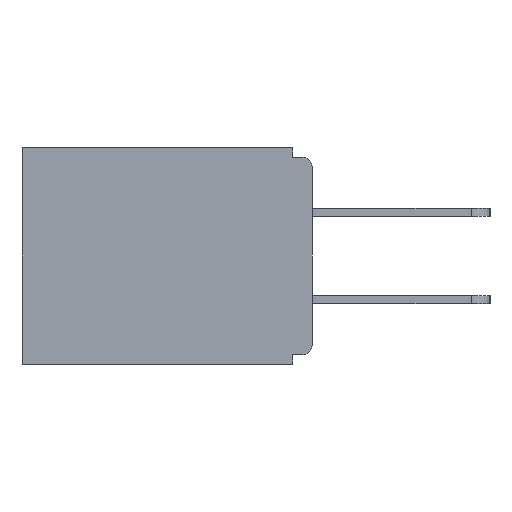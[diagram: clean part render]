
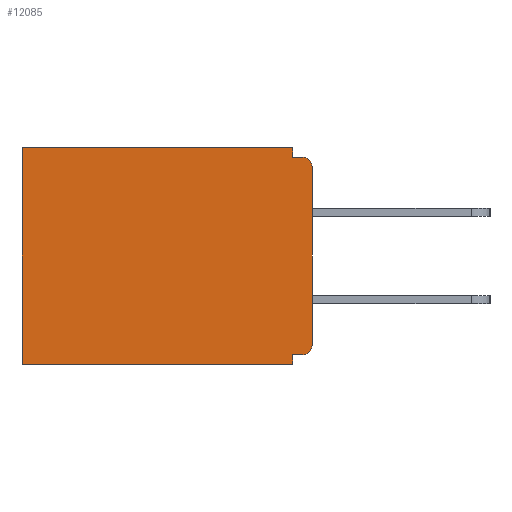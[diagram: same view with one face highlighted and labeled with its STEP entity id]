
A CAD part, left-side view. The second image highlights one B-rep face of the part: STEP entity #12085.
In plain terms, the highlighted planar face has unit normal (-1, 0, 0).
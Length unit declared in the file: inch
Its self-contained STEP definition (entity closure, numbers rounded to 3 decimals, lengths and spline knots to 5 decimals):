
#269 = ORIENTED_EDGE ( 'NONE', *, *, #14848, .F. ) ;
#725 = AXIS2_PLACEMENT_3D ( 'NONE', #785, #15022, #5420 ) ;
#785 = CARTESIAN_POINT ( 'NONE',  ( 0.298, 0.015, -0.03 ) ) ;
#823 = VECTOR ( 'NONE', #6712, 39.37008 ) ;
#898 = EDGE_CURVE ( 'NONE', #6197, #3613, #15210, .T. ) ;
#1183 = LINE ( 'NONE', #10388, #823 ) ;
#1214 = EDGE_CURVE ( 'NONE', #7799, #14307, #14885, .T. ) ;
#1244 = ORIENTED_EDGE ( 'NONE', *, *, #13400, .F. ) ;
#1270 = AXIS2_PLACEMENT_3D ( 'NONE', #12982, #9549, #7104 ) ;
#1439 = DIRECTION ( 'NONE',  ( 0., 0., -1. ) ) ;
#1534 = VERTEX_POINT ( 'NONE', #3962 ) ;
#1569 = EDGE_LOOP ( 'NONE', ( #6287, #1244, #14124, #11355, #6634, #13552, #6143, #15362, #12694, #269 ) ) ;
#1958 = VERTEX_POINT ( 'NONE', #3737 ) ;
#2016 = DIRECTION ( 'NONE',  ( 0., 0., -1. ) ) ;
#2273 = CARTESIAN_POINT ( 'NONE',  ( 0.298, 0.46, 0. ) ) ;
#2879 = EDGE_CURVE ( 'NONE', #6197, #12429, #9431, .T. ) ;
#2928 = LINE ( 'NONE', #14423, #4573 ) ;
#3182 = DIRECTION ( 'NONE',  ( 0., 1., 0. ) ) ;
#3613 = VERTEX_POINT ( 'NONE', #11995 ) ;
#3727 = CARTESIAN_POINT ( 'NONE',  ( 0.298, 0.015, -0.313 ) ) ;
#3737 = CARTESIAN_POINT ( 'NONE',  ( 0.298, 0., -0.313 ) ) ;
#3962 = CARTESIAN_POINT ( 'NONE',  ( 0.298, 0., -0.03 ) ) ;
#4268 = CARTESIAN_POINT ( 'NONE',  ( 0.298, 0.031, -0.328 ) ) ;
#4573 = VECTOR ( 'NONE', #7696, 39.37008 ) ;
#4644 = EDGE_CURVE ( 'NONE', #5984, #1958, #10282, .T. ) ;
#4909 = DIRECTION ( 'NONE',  ( -1., 0., 0. ) ) ;
#5175 = DIRECTION ( 'NONE',  ( 0., 1., 0. ) ) ;
#5420 = DIRECTION ( 'NONE',  ( 0., 0., -1. ) ) ;
#5594 = CARTESIAN_POINT ( 'NONE',  ( 0.298, 0., -0.328 ) ) ;
#5964 = CARTESIAN_POINT ( 'NONE',  ( 0.298, 0.031, -0.343 ) ) ;
#5984 = VERTEX_POINT ( 'NONE', #12287 ) ;
#6143 = ORIENTED_EDGE ( 'NONE', *, *, #15370, .F. ) ;
#6197 = VERTEX_POINT ( 'NONE', #10398 ) ;
#6287 = ORIENTED_EDGE ( 'NONE', *, *, #13586, .T. ) ;
#6634 = ORIENTED_EDGE ( 'NONE', *, *, #12785, .T. ) ;
#6712 = DIRECTION ( 'NONE',  ( 0., 0., -1. ) ) ;
#6801 = CARTESIAN_POINT ( 'NONE',  ( 0.298, 0.031, -0.343 ) ) ;
#7104 = DIRECTION ( 'NONE',  ( 0., 0., -1. ) ) ;
#7174 = LINE ( 'NONE', #6801, #12936 ) ;
#7478 = CARTESIAN_POINT ( 'NONE',  ( 0.298, 0., 0. ) ) ;
#7532 = DIRECTION ( 'NONE',  ( 0., 1., 0. ) ) ;
#7696 = DIRECTION ( 'NONE',  ( 0., -1., 0. ) ) ;
#7799 = VERTEX_POINT ( 'NONE', #10192 ) ;
#8160 = CIRCLE ( 'NONE', #725, 0.015 ) ;
#8318 = VECTOR ( 'NONE', #7532, 39.37008 ) ;
#8502 = VECTOR ( 'NONE', #3182, 39.37008 ) ;
#8692 = FACE_OUTER_BOUND ( 'NONE', #1569, .T. ) ;
#9431 = LINE ( 'NONE', #7478, #8318 ) ;
#9549 = DIRECTION ( 'NONE',  ( 1., 0., 0. ) ) ;
#9688 = DIRECTION ( 'NONE',  ( 0., 0., -1. ) ) ;
#10192 = CARTESIAN_POINT ( 'NONE',  ( 0.298, 0.031, -0.343 ) ) ;
#10282 = CIRCLE ( 'NONE', #15294, 0.015 ) ;
#10388 = CARTESIAN_POINT ( 'NONE',  ( 0.298, 0.46, 0. ) ) ;
#10398 = CARTESIAN_POINT ( 'NONE',  ( 0.298, 0.031, 0. ) ) ;
#10576 = VECTOR ( 'NONE', #5175, 39.37008 ) ;
#11006 = CARTESIAN_POINT ( 'NONE',  ( 0.298, 0.015, -0.015 ) ) ;
#11272 = VECTOR ( 'NONE', #9688, 39.37008 ) ;
#11355 = ORIENTED_EDGE ( 'NONE', *, *, #2879, .T. ) ;
#11772 = PLANE ( 'NONE',  #1270 ) ;
#11795 = DIRECTION ( 'NONE',  ( 0., 0., -1. ) ) ;
#11995 = CARTESIAN_POINT ( 'NONE',  ( 0.298, 0.031, -0.015 ) ) ;
#12019 = VECTOR ( 'NONE', #11795, 39.37008 ) ;
#12085 = ADVANCED_FACE ( 'NONE', ( #8692 ), #11772, .F. ) ;
#12116 = CARTESIAN_POINT ( 'NONE',  ( 0.298, 0., 0. ) ) ;
#12136 = CARTESIAN_POINT ( 'NONE',  ( 0.298, 0.46, -0.343 ) ) ;
#12195 = LINE ( 'NONE', #5594, #8502 ) ;
#12287 = CARTESIAN_POINT ( 'NONE',  ( 0.298, 0.015, -0.328 ) ) ;
#12429 = VERTEX_POINT ( 'NONE', #2273 ) ;
#12694 = ORIENTED_EDGE ( 'NONE', *, *, #4644, .T. ) ;
#12764 = EDGE_CURVE ( 'NONE', #5984, #15315, #12195, .T. ) ;
#12785 = EDGE_CURVE ( 'NONE', #12429, #14307, #1183, .T. ) ;
#12936 = VECTOR ( 'NONE', #2016, 39.37008 ) ;
#12982 = CARTESIAN_POINT ( 'NONE',  ( 0.298, 0., 0. ) ) ;
#13400 = EDGE_CURVE ( 'NONE', #3613, #15242, #2928, .T. ) ;
#13552 = ORIENTED_EDGE ( 'NONE', *, *, #1214, .F. ) ;
#13586 = EDGE_CURVE ( 'NONE', #1534, #15242, #8160, .T. ) ;
#13735 = CARTESIAN_POINT ( 'NONE',  ( 0.298, 0., -0.343 ) ) ;
#14124 = ORIENTED_EDGE ( 'NONE', *, *, #898, .F. ) ;
#14307 = VERTEX_POINT ( 'NONE', #12136 ) ;
#14423 = CARTESIAN_POINT ( 'NONE',  ( 0.298, 0., -0.015 ) ) ;
#14848 = EDGE_CURVE ( 'NONE', #1534, #1958, #15002, .T. ) ;
#14885 = LINE ( 'NONE', #13735, #10576 ) ;
#15002 = LINE ( 'NONE', #12116, #11272 ) ;
#15022 = DIRECTION ( 'NONE',  ( -1., 0., 0. ) ) ;
#15210 = LINE ( 'NONE', #5964, #12019 ) ;
#15242 = VERTEX_POINT ( 'NONE', #11006 ) ;
#15294 = AXIS2_PLACEMENT_3D ( 'NONE', #3727, #4909, #1439 ) ;
#15315 = VERTEX_POINT ( 'NONE', #4268 ) ;
#15362 = ORIENTED_EDGE ( 'NONE', *, *, #12764, .F. ) ;
#15370 = EDGE_CURVE ( 'NONE', #15315, #7799, #7174, .T. ) ;
